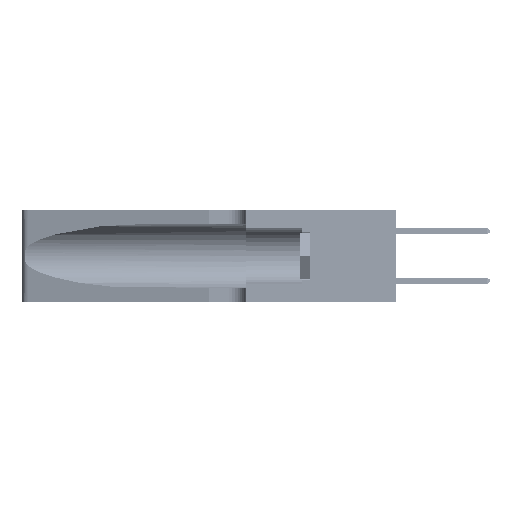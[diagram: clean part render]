
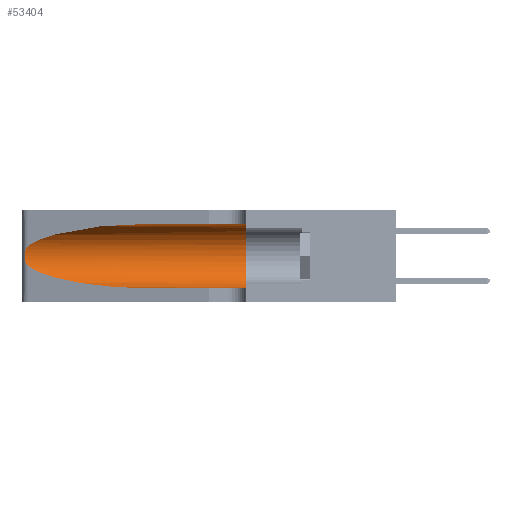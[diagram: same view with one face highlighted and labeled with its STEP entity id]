
A CAD part, left-side view. The second image highlights one B-rep face of the part: STEP entity #53404.
In plain terms, the highlighted cylindrical face has radius 3.308 mm (diameter 6.617 mm), a partial arc.
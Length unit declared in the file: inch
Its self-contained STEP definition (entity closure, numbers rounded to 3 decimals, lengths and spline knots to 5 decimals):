
#709 = CARTESIAN_POINT ( 'NONE',  ( 0.1305, 0.72297, 0.05475 ) ) ;
#1326 = VECTOR ( 'NONE', #28254, 39.37008 ) ;
#1426 = ORIENTED_EDGE ( 'NONE', *, *, #10060, .T. ) ;
#1430 = EDGE_LOOP ( 'NONE', ( #20443, #44873, #14653, #1426, #11512, #41077 ) ) ;
#1524 = CARTESIAN_POINT ( 'NONE',  ( 0.1305, 1.61858, 0.31525 ) ) ;
#1582 = CARTESIAN_POINT ( 'NONE',  ( 0.25787, 1.23484, 0.2124 ) ) ;
#3046 = CARTESIAN_POINT ( 'NONE',  ( 0.1305, 1.61858, 0.05475 ) ) ;
#3273 = DIRECTION ( 'NONE',  ( 0., 1., 0. ) ) ;
#5871 = CARTESIAN_POINT ( 'NONE',  ( 0.26018, 1.23835, 0.19895 ) ) ;
#7227 = CIRCLE ( 'NONE', #52836, 0.13025 ) ;
#9367 =( BOUNDED_CURVE ( )  B_SPLINE_CURVE ( 3, ( #34141, #46599, #25944, #709 ),
 .UNSPECIFIED., .F., .F. ) 
 B_SPLINE_CURVE_WITH_KNOTS ( ( 4, 4 ),
 ( 3.44316, 4.71239 ),
 .UNSPECIFIED. ) 
 CURVE ( )  GEOMETRIC_REPRESENTATION_ITEM ( )  RATIONAL_B_SPLINE_CURVE ( ( 1., 0.87, 0.87, 1. ) ) 
 REPRESENTATION_ITEM ( '' )  );
#10060 = EDGE_CURVE ( 'NONE', #36218, #40895, #23743, .T. ) ;
#10080 = DIRECTION ( 'NONE',  ( 0., -1., 0. ) ) ;
#10140 = CARTESIAN_POINT ( 'NONE',  ( 0.26075, 1.23896, 0.178 ) ) ;
#11512 = ORIENTED_EDGE ( 'NONE', *, *, #49631, .F. ) ;
#13357 = DIRECTION ( 'NONE',  ( 0., 0., -1. ) ) ;
#14174 = CARTESIAN_POINT ( 'NONE',  ( 0.25555, 1.22994, 0.2215 ) ) ;
#14352 = CARTESIAN_POINT ( 'NONE',  ( 0.25856, 1.23593, 0.16098 ) ) ;
#14653 = ORIENTED_EDGE ( 'NONE', *, *, #47363, .T. ) ;
#18570 = CARTESIAN_POINT ( 'NONE',  ( 0.25639, 1.23186, 0.15144 ) ) ;
#19079 = FACE_OUTER_BOUND ( 'NONE', #1430, .T. ) ;
#19326 = CARTESIAN_POINT ( 'NONE',  ( 0.2373, 1.15595, 0.28018 ) ) ;
#20443 = ORIENTED_EDGE ( 'NONE', *, *, #35690, .T. ) ;
#22782 = CARTESIAN_POINT ( 'NONE',  ( 0.25487, 1.22718, 0.14631 ) ) ;
#23343 = VERTEX_POINT ( 'NONE', #36984 ) ;
#23372 = CARTESIAN_POINT ( 'NONE',  ( 0.18966, 0.96281, 0.31525 ) ) ;
#23743 = LINE ( 'NONE', #3046, #1326 ) ;
#24528 = CARTESIAN_POINT ( 'NONE',  ( 0.1305, 0.72297, 0.31525 ) ) ;
#25944 = CARTESIAN_POINT ( 'NONE',  ( 0.18966, 0.96281, 0.05475 ) ) ;
#26825 = CARTESIAN_POINT ( 'NONE',  ( 0.25639, 1.23184, 0.21858 ) ) ;
#27516 = CARTESIAN_POINT ( 'NONE',  ( 0.1305, 0.35, 0.31525 ) ) ;
#27738 = CARTESIAN_POINT ( 'NONE',  ( 0.1305, 0.72297, 0.05475 ) ) ;
#28254 = DIRECTION ( 'NONE',  ( 0., -1., 0. ) ) ;
#28472 = CARTESIAN_POINT ( 'NONE',  ( 0.1305, 0.35, 0.185 ) ) ;
#31029 = CARTESIAN_POINT ( 'NONE',  ( 0.25854, 1.2359, 0.20912 ) ) ;
#31819 = VERTEX_POINT ( 'NONE', #42513 ) ;
#32644 = DIRECTION ( 'NONE',  ( 0., 0., 1. ) ) ;
#34141 = CARTESIAN_POINT ( 'NONE',  ( 0.25487, 1.22718, 0.14631 ) ) ;
#34184 = DIRECTION ( 'NONE',  ( 0., -1., 0. ) ) ;
#35190 = CARTESIAN_POINT ( 'NONE',  ( 0.26075, 1.23896, 0.19203 ) ) ;
#35690 = EDGE_CURVE ( 'NONE', #40159, #23343, #38485, .T. ) ;
#36218 = VERTEX_POINT ( 'NONE', #27738 ) ;
#36752 = EDGE_CURVE ( 'NONE', #40159, #48132, #41417, .T. ) ;
#36984 = CARTESIAN_POINT ( 'NONE',  ( 0.25487, 1.22718, 0.22369 ) ) ;
#38332 = CARTESIAN_POINT ( 'NONE',  ( 0.1305, 1.61858, 0.185 ) ) ;
#38485 =( BOUNDED_CURVE ( )  B_SPLINE_CURVE ( 3, ( #52175, #23372, #19326, #48370 ),
 .UNSPECIFIED., .F., .F. ) 
 B_SPLINE_CURVE_WITH_KNOTS ( ( 4, 4 ),
 ( 1.5708, 2.84003 ),
 .UNSPECIFIED. ) 
 CURVE ( )  GEOMETRIC_REPRESENTATION_ITEM ( )  RATIONAL_B_SPLINE_CURVE ( ( 1., 0.87, 0.87, 1. ) ) 
 REPRESENTATION_ITEM ( '' )  );
#39333 = CARTESIAN_POINT ( 'NONE',  ( 0.26017, 1.23833, 0.17102 ) ) ;
#40159 = VERTEX_POINT ( 'NONE', #24528 ) ;
#40895 = VERTEX_POINT ( 'NONE', #45672 ) ;
#41077 = ORIENTED_EDGE ( 'NONE', *, *, #36752, .F. ) ;
#41417 = LINE ( 'NONE', #1524, #51062 ) ;
#42513 = CARTESIAN_POINT ( 'NONE',  ( 0.25487, 1.22718, 0.14631 ) ) ;
#43309 = CARTESIAN_POINT ( 'NONE',  ( 0.25487, 1.22718, 0.22369 ) ) ;
#43486 = CARTESIAN_POINT ( 'NONE',  ( 0.25789, 1.23486, 0.15765 ) ) ;
#44319 = AXIS2_PLACEMENT_3D ( 'NONE', #38332, #34184, #13357 ) ;
#44873 = ORIENTED_EDGE ( 'NONE', *, *, #52356, .T. ) ;
#45672 = CARTESIAN_POINT ( 'NONE',  ( 0.1305, 0.35, 0.05475 ) ) ;
#46599 = CARTESIAN_POINT ( 'NONE',  ( 0.2373, 1.15595, 0.08982 ) ) ;
#47363 = EDGE_CURVE ( 'NONE', #31819, #36218, #9367, .T. ) ;
#47615 = CARTESIAN_POINT ( 'NONE',  ( 0.25555, 1.22993, 0.14849 ) ) ;
#48132 = VERTEX_POINT ( 'NONE', #27516 ) ;
#48370 = CARTESIAN_POINT ( 'NONE',  ( 0.25487, 1.22718, 0.22369 ) ) ;
#49631 = EDGE_CURVE ( 'NONE', #48132, #40895, #7227, .T. ) ;
#50882 = CYLINDRICAL_SURFACE ( 'NONE', #44319, 0.13025 ) ;
#51062 = VECTOR ( 'NONE', #10080, 39.37008 ) ;
#52175 = CARTESIAN_POINT ( 'NONE',  ( 0.1305, 0.72297, 0.31525 ) ) ;
#52356 = EDGE_CURVE ( 'NONE', #23343, #31819, #53667, .T. ) ;
#52836 = AXIS2_PLACEMENT_3D ( 'NONE', #28472, #3273, #32644 ) ;
#53404 = ADVANCED_FACE ( 'NONE', ( #19079 ), #50882, .F. ) ;
#53667 = B_SPLINE_CURVE_WITH_KNOTS ( 'NONE', 3,
 ( #43309, #14174, #26825, #1582, #31029, #5871, #35190, #10140, #39333, #14352, #43486, #18570, #47615, #22782 ),
 .UNSPECIFIED., .F., .F.,
 ( 4, 2, 2, 2, 2, 2, 4 ),
 ( 0., 0.00027, 0.00053, 0.00107, 0.0016, 0.00187, 0.00214 ),
 .UNSPECIFIED. ) ;
